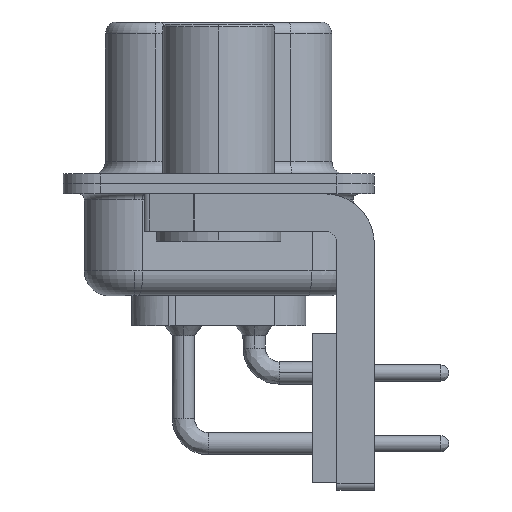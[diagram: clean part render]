
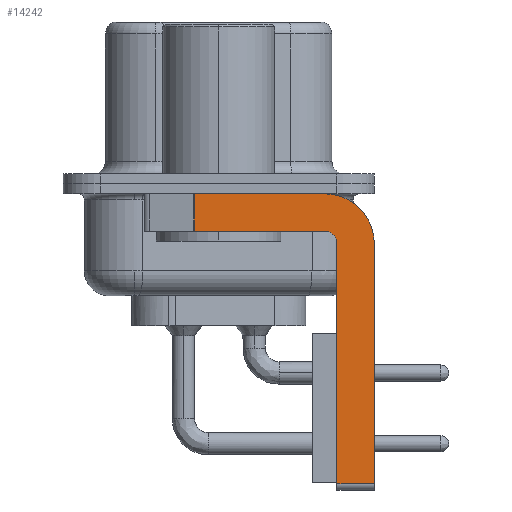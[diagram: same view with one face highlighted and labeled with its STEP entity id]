
A CAD part, left-side view. The second image highlights one B-rep face of the part: STEP entity #14242.
In plain terms, the highlighted planar face has unit normal (-1, 0, 0).
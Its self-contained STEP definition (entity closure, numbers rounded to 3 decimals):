
#392 = VECTOR ( 'NONE', #12322, 1000. ) ;
#446 = DIRECTION ( 'NONE',  ( 0., 0., -1. ) ) ;
#817 = EDGE_CURVE ( 'NONE', #3493, #9452, #15206, .T. ) ;
#1078 = ORIENTED_EDGE ( 'NONE', *, *, #6786, .T. ) ;
#1320 = CARTESIAN_POINT ( 'NONE',  ( -2.9, 3., -0.4 ) ) ;
#1371 = DIRECTION ( 'NONE',  ( 0., -1., 0. ) ) ;
#1504 = ORIENTED_EDGE ( 'NONE', *, *, #21577, .T. ) ;
#1827 = CARTESIAN_POINT ( 'NONE',  ( -2.9, -6.25, -2.4 ) ) ;
#1895 = EDGE_CURVE ( 'NONE', #23806, #2310, #2731, .T. ) ;
#2310 = VERTEX_POINT ( 'NONE', #19013 ) ;
#2731 = LINE ( 'NONE', #1320, #17888 ) ;
#2733 = DIRECTION ( 'NONE',  ( 0., 0., 1. ) ) ;
#3493 = VERTEX_POINT ( 'NONE', #1827 ) ;
#3656 = EDGE_CURVE ( 'NONE', #2310, #3493, #4236, .T. ) ;
#3981 = VECTOR ( 'NONE', #10212, 1000. ) ;
#4236 = CIRCLE ( 'NONE', #24511, 2. ) ;
#4330 = VERTEX_POINT ( 'NONE', #13724 ) ;
#4360 = PLANE ( 'NONE',  #18088 ) ;
#4608 = DIRECTION ( 'NONE',  ( 0., 0., -1. ) ) ;
#4946 = DIRECTION ( 'NONE',  ( 1., 0., 0. ) ) ;
#5212 = CARTESIAN_POINT ( 'NONE',  ( -2.9, -4.25, -2.4 ) ) ;
#5455 = ORIENTED_EDGE ( 'NONE', *, *, #1895, .F. ) ;
#6221 = CARTESIAN_POINT ( 'NONE',  ( -2.9, -6.25, -12.05 ) ) ;
#6306 = LINE ( 'NONE', #20647, #22603 ) ;
#6380 = CARTESIAN_POINT ( 'NONE',  ( -2.9, -4.25, -2.4 ) ) ;
#6638 = VECTOR ( 'NONE', #22255, 1000. ) ;
#6786 = EDGE_CURVE ( 'NONE', #23806, #20356, #12560, .T. ) ;
#7132 = EDGE_CURVE ( 'NONE', #4330, #18137, #21165, .T. ) ;
#7937 = EDGE_CURVE ( 'NONE', #18137, #20356, #16139, .T. ) ;
#8218 = CARTESIAN_POINT ( 'NONE',  ( -2.9, -4.25, -12.05 ) ) ;
#8327 = DIRECTION ( 'NONE',  ( 0., 0., 1. ) ) ;
#9092 = CARTESIAN_POINT ( 'NONE',  ( -2.9, -4.25, -2.4 ) ) ;
#9282 = AXIS2_PLACEMENT_3D ( 'NONE', #9092, #9434, #8327 ) ;
#9283 = LINE ( 'NONE', #8218, #3981 ) ;
#9434 = DIRECTION ( 'NONE',  ( -1., 0., 0. ) ) ;
#9452 = VERTEX_POINT ( 'NONE', #6221 ) ;
#10212 = DIRECTION ( 'NONE',  ( 0., -1., 0. ) ) ;
#10300 = CARTESIAN_POINT ( 'NONE',  ( -2.9, -4.25, -1.9 ) ) ;
#11964 = ORIENTED_EDGE ( 'NONE', *, *, #817, .F. ) ;
#12322 = DIRECTION ( 'NONE',  ( 0., 1., 0. ) ) ;
#12371 = DIRECTION ( 'NONE',  ( 1., 0., 0. ) ) ;
#12560 = LINE ( 'NONE', #20981, #6638 ) ;
#12586 = VERTEX_POINT ( 'NONE', #22812 ) ;
#13175 = FACE_OUTER_BOUND ( 'NONE', #15887, .T. ) ;
#13724 = CARTESIAN_POINT ( 'NONE',  ( -2.9, -4.75, -2.4 ) ) ;
#14242 = ADVANCED_FACE ( 'NONE', ( #13175 ), #4360, .F. ) ;
#15100 = CARTESIAN_POINT ( 'NONE',  ( -2.9, 0.978, -0.4 ) ) ;
#15206 = LINE ( 'NONE', #20321, #25023 ) ;
#15887 = EDGE_LOOP ( 'NONE', ( #5455, #1078, #21076, #24996, #22944, #1504, #11964, #21870 ) ) ;
#16139 = LINE ( 'NONE', #10300, #392 ) ;
#16609 = CARTESIAN_POINT ( 'NONE',  ( -2.9, -4.25, -1.9 ) ) ;
#17888 = VECTOR ( 'NONE', #1371, 1000. ) ;
#18088 = AXIS2_PLACEMENT_3D ( 'NONE', #6380, #12371, #446 ) ;
#18137 = VERTEX_POINT ( 'NONE', #16609 ) ;
#19013 = CARTESIAN_POINT ( 'NONE',  ( -2.9, -4.25, -0.4 ) ) ;
#19293 = EDGE_CURVE ( 'NONE', #12586, #4330, #6306, .T. ) ;
#19905 = DIRECTION ( 'NONE',  ( 0., 0., -1. ) ) ;
#20321 = CARTESIAN_POINT ( 'NONE',  ( -2.9, -6.25, -2.4 ) ) ;
#20356 = VERTEX_POINT ( 'NONE', #24175 ) ;
#20647 = CARTESIAN_POINT ( 'NONE',  ( -2.9, -4.75, -12.3 ) ) ;
#20981 = CARTESIAN_POINT ( 'NONE',  ( -2.9, 0.978, -1.9 ) ) ;
#21076 = ORIENTED_EDGE ( 'NONE', *, *, #7937, .F. ) ;
#21165 = CIRCLE ( 'NONE', #9282, 0.5 ) ;
#21577 = EDGE_CURVE ( 'NONE', #12586, #9452, #9283, .T. ) ;
#21870 = ORIENTED_EDGE ( 'NONE', *, *, #3656, .F. ) ;
#22255 = DIRECTION ( 'NONE',  ( 0., 0., -1. ) ) ;
#22603 = VECTOR ( 'NONE', #2733, 1000. ) ;
#22812 = CARTESIAN_POINT ( 'NONE',  ( -2.9, -4.75, -12.05 ) ) ;
#22944 = ORIENTED_EDGE ( 'NONE', *, *, #19293, .F. ) ;
#23806 = VERTEX_POINT ( 'NONE', #15100 ) ;
#24175 = CARTESIAN_POINT ( 'NONE',  ( -2.9, 0.978, -1.9 ) ) ;
#24511 = AXIS2_PLACEMENT_3D ( 'NONE', #5212, #4946, #4608 ) ;
#24996 = ORIENTED_EDGE ( 'NONE', *, *, #7132, .F. ) ;
#25023 = VECTOR ( 'NONE', #19905, 1000. ) ;
